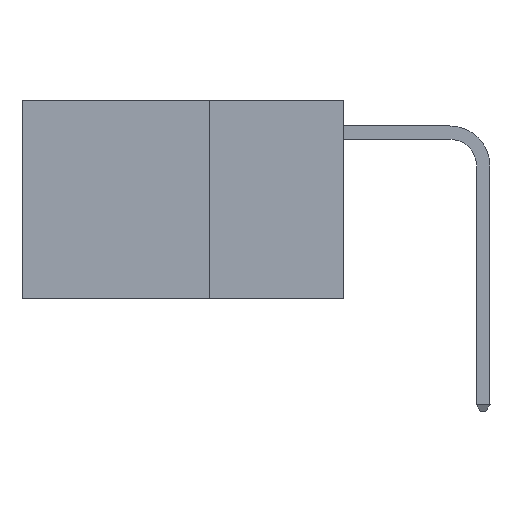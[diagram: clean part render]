
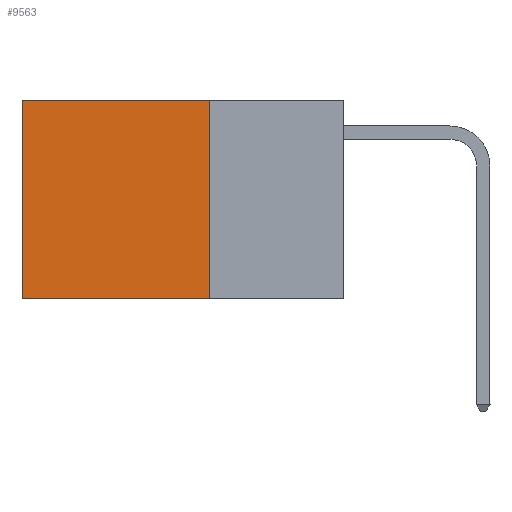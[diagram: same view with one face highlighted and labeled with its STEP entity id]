
A CAD part, left-side view. The second image highlights one B-rep face of the part: STEP entity #9563.
In plain terms, the highlighted planar face has unit normal (-1, 0, 0).
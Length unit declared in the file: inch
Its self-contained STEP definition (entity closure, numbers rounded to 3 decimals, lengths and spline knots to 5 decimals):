
#293 = CARTESIAN_POINT ( 'NONE',  ( 0.2625, 0.25, 0. ) ) ;
#438 = EDGE_CURVE ( 'NONE', #12126, #3833, #504, .T. ) ;
#504 = LINE ( 'NONE', #12099, #548 ) ;
#548 = VECTOR ( 'NONE', #7117, 39.37008 ) ;
#554 = CARTESIAN_POINT ( 'NONE',  ( 0.2625, 0.25, 0. ) ) ;
#2530 = VERTEX_POINT ( 'NONE', #2537 ) ;
#2537 = CARTESIAN_POINT ( 'NONE',  ( 0.2625, 0.25, -0.37 ) ) ;
#2662 = LINE ( 'NONE', #3166, #5159 ) ;
#3166 = CARTESIAN_POINT ( 'NONE',  ( 0.2625, 0.25, 0. ) ) ;
#3532 = FACE_OUTER_BOUND ( 'NONE', #7438, .T. ) ;
#3823 = EDGE_CURVE ( 'NONE', #2530, #3833, #8456, .T. ) ;
#3833 = VERTEX_POINT ( 'NONE', #8169 ) ;
#4498 = DIRECTION ( 'NONE',  ( 0., 1., 0. ) ) ;
#4746 = VERTEX_POINT ( 'NONE', #293 ) ;
#4885 = DIRECTION ( 'NONE',  ( 1., 0., 0. ) ) ;
#5066 = LINE ( 'NONE', #11606, #5399 ) ;
#5159 = VECTOR ( 'NONE', #12349, 39.37008 ) ;
#5399 = VECTOR ( 'NONE', #4498, 39.37008 ) ;
#5719 = VECTOR ( 'NONE', #8187, 39.37008 ) ;
#7117 = DIRECTION ( 'NONE',  ( 0., 0., -1. ) ) ;
#7199 = ORIENTED_EDGE ( 'NONE', *, *, #438, .T. ) ;
#7438 = EDGE_LOOP ( 'NONE', ( #7199, #8240, #8767, #9593 ) ) ;
#8169 = CARTESIAN_POINT ( 'NONE',  ( 0.2625, 0.6, -0.37 ) ) ;
#8187 = DIRECTION ( 'NONE',  ( 0., 1., 0. ) ) ;
#8240 = ORIENTED_EDGE ( 'NONE', *, *, #3823, .F. ) ;
#8263 = CARTESIAN_POINT ( 'NONE',  ( 0.2625, 0.25, -0.37 ) ) ;
#8456 = LINE ( 'NONE', #8263, #5719 ) ;
#8767 = ORIENTED_EDGE ( 'NONE', *, *, #9823, .F. ) ;
#8992 = PLANE ( 'NONE',  #10996 ) ;
#9563 = ADVANCED_FACE ( 'NONE', ( #3532 ), #8992, .F. ) ;
#9593 = ORIENTED_EDGE ( 'NONE', *, *, #12816, .T. ) ;
#9823 = EDGE_CURVE ( 'NONE', #4746, #2530, #2662, .T. ) ;
#10996 = AXIS2_PLACEMENT_3D ( 'NONE', #554, #4885, #11965 ) ;
#11606 = CARTESIAN_POINT ( 'NONE',  ( 0.2625, 0.25, 0. ) ) ;
#11965 = DIRECTION ( 'NONE',  ( 0., 0., -1. ) ) ;
#12099 = CARTESIAN_POINT ( 'NONE',  ( 0.2625, 0.6, 0. ) ) ;
#12126 = VERTEX_POINT ( 'NONE', #12959 ) ;
#12349 = DIRECTION ( 'NONE',  ( 0., 0., -1. ) ) ;
#12816 = EDGE_CURVE ( 'NONE', #4746, #12126, #5066, .T. ) ;
#12959 = CARTESIAN_POINT ( 'NONE',  ( 0.2625, 0.6, 0. ) ) ;
